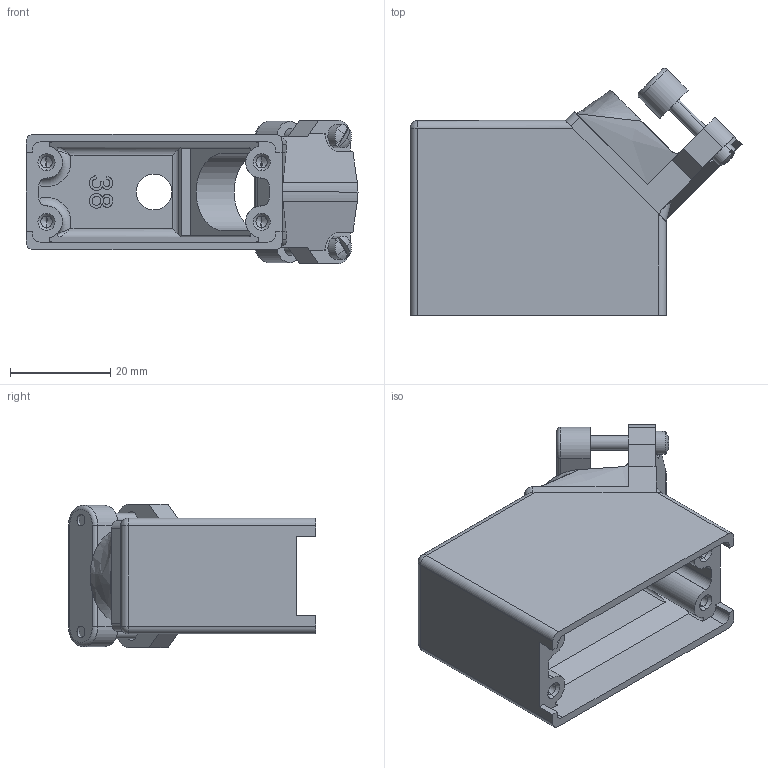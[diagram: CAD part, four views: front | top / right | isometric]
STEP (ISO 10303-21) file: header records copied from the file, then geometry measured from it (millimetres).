
FILE_DESCRIPTION (( 'STEP AP203' ), '1' );
FILE_NAME ('516-230-738.STEP', '2021-05-13T18:14:54', ( '' ), ( '' ), 'SwSTEP 2.0', 'SolidWorks 2020', '' );
FILE_SCHEMA (( 'CONFIG_CONTROL_DESIGN' ));
Length unit declared in the file: inch
Products named in the file (6): 516-231-341; 516-230-738; 516-231-007_516-231-042; PLASTIC BODY; fillister head screw_ai_4-40 UNC-2A; 516-230-038_516-230-042
Assembly tree (6 placements, depth 3):
  516-230-738
    PLASTIC BODY
      516-230-038_516-230-042
      516-231-341
    516-231-007_516-231-042
    fillister head screw_ai_4-40 UNC-2A  x2
Bounding box: 66.18 x 49.24 x 28.57 mm (x, y, z)
Volume: 19283.5 mm3; surface area: 15606.7 mm2
Topology: 5 solids, 5 shells, 360 faces, 964 edges, 624 vertices
Faces by surface type: plane 159, bspline 79, cylinder 78, cone 28, sphere 12, torus 4
Entity records: 15868 total; most frequent: CARTESIAN_POINT 7072, ORIENTED_EDGE 1844, DIRECTION 1434, EDGE_CURVE 922, VERTEX_POINT 604, LINE 550, VECTOR 550, AXIS2_PLACEMENT_3D 442
